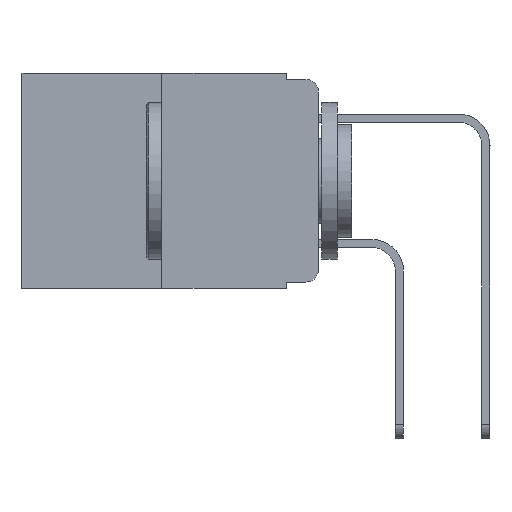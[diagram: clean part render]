
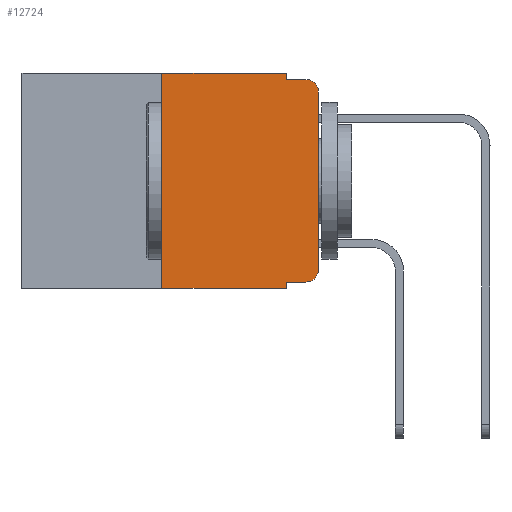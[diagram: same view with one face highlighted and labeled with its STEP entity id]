
A CAD part, left-side view. The second image highlights one B-rep face of the part: STEP entity #12724.
In plain terms, the highlighted planar face has unit normal (-1, 0, 0).
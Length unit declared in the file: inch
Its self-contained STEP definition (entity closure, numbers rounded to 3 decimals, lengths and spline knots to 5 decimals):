
#627 = LINE ( 'NONE', #11307, #21757 ) ;
#1274 = VERTEX_POINT ( 'NONE', #8650 ) ;
#1447 = VECTOR ( 'NONE', #20146, 39.37008 ) ;
#1574 = EDGE_CURVE ( 'NONE', #1274, #16716, #19780, .T. ) ;
#1789 = ORIENTED_EDGE ( 'NONE', *, *, #14009, .F. ) ;
#2052 = FACE_OUTER_BOUND ( 'NONE', #8509, .T. ) ;
#2379 = DIRECTION ( 'NONE',  ( 0., -1., 0. ) ) ;
#2404 = VECTOR ( 'NONE', #9807, 39.37008 ) ;
#2467 = LINE ( 'NONE', #9167, #5246 ) ;
#3691 = VERTEX_POINT ( 'NONE', #8519 ) ;
#4046 = VECTOR ( 'NONE', #21586, 39.37008 ) ;
#4500 = VECTOR ( 'NONE', #20394, 39.37008 ) ;
#4790 = VERTEX_POINT ( 'NONE', #8378 ) ;
#4875 = CARTESIAN_POINT ( 'NONE',  ( 0., 0.25, 0. ) ) ;
#5116 = ORIENTED_EDGE ( 'NONE', *, *, #1574, .T. ) ;
#5246 = VECTOR ( 'NONE', #16321, 39.37008 ) ;
#5424 = ORIENTED_EDGE ( 'NONE', *, *, #16774, .T. ) ;
#5484 = CARTESIAN_POINT ( 'NONE',  ( 0., 0.02, -0.03 ) ) ;
#6017 = LINE ( 'NONE', #20479, #2404 ) ;
#6065 = CARTESIAN_POINT ( 'NONE',  ( 0., 0.02, -0.333 ) ) ;
#6272 = VECTOR ( 'NONE', #22217, 39.37008 ) ;
#7768 = AXIS2_PLACEMENT_3D ( 'NONE', #10038, #13633, #17211 ) ;
#7793 = CARTESIAN_POINT ( 'NONE',  ( 0., 0.473, -0.343 ) ) ;
#8199 = LINE ( 'NONE', #14960, #6272 ) ;
#8378 = CARTESIAN_POINT ( 'NONE',  ( 0., 0.051, 0. ) ) ;
#8495 = CARTESIAN_POINT ( 'NONE',  ( 0., 0.051, -0.343 ) ) ;
#8509 = EDGE_LOOP ( 'NONE', ( #22162, #5424, #14634, #11281, #1789, #23008, #5116, #17263, #17312, #12977 ) ) ;
#8519 = CARTESIAN_POINT ( 'NONE',  ( 0., 0., -0.313 ) ) ;
#8650 = CARTESIAN_POINT ( 'NONE',  ( 0., 0.25, -0.343 ) ) ;
#8924 = LINE ( 'NONE', #17267, #1447 ) ;
#9161 = CARTESIAN_POINT ( 'NONE',  ( 0., 0.051, -0.01 ) ) ;
#9167 = CARTESIAN_POINT ( 'NONE',  ( 0., 0.051, -0.333 ) ) ;
#9543 = EDGE_CURVE ( 'NONE', #1274, #20126, #17157, .T. ) ;
#9807 = DIRECTION ( 'NONE',  ( 0., 0., 1. ) ) ;
#10038 = CARTESIAN_POINT ( 'NONE',  ( 0., 0.02, -0.313 ) ) ;
#10451 = CIRCLE ( 'NONE', #22774, 0.02 ) ;
#10657 = LINE ( 'NONE', #12635, #4046 ) ;
#10987 = EDGE_CURVE ( 'NONE', #13786, #16716, #10657, .T. ) ;
#11281 = ORIENTED_EDGE ( 'NONE', *, *, #17051, .F. ) ;
#11307 = CARTESIAN_POINT ( 'NONE',  ( 0., 0.051, -0.01 ) ) ;
#11659 = EDGE_CURVE ( 'NONE', #13728, #3691, #20128, .T. ) ;
#11779 = CARTESIAN_POINT ( 'NONE',  ( 0., 0.02, -0.01 ) ) ;
#12148 = VECTOR ( 'NONE', #13687, 39.37008 ) ;
#12386 = DIRECTION ( 'NONE',  ( 0., 0., -1. ) ) ;
#12558 = CARTESIAN_POINT ( 'NONE',  ( 0., 0.051, -0.333 ) ) ;
#12615 = DIRECTION ( 'NONE',  ( -1., 0., 0. ) ) ;
#12635 = CARTESIAN_POINT ( 'NONE',  ( 0., 0.051, 0. ) ) ;
#12724 = ADVANCED_FACE ( 'NONE', ( #2052 ), #13931, .F. ) ;
#12977 = ORIENTED_EDGE ( 'NONE', *, *, #11659, .T. ) ;
#13442 = AXIS2_PLACEMENT_3D ( 'NONE', #22747, #19292, #19154 ) ;
#13633 = DIRECTION ( 'NONE',  ( -1., 0., 0. ) ) ;
#13687 = DIRECTION ( 'NONE',  ( 0., 0., 1. ) ) ;
#13728 = VERTEX_POINT ( 'NONE', #6065 ) ;
#13786 = VERTEX_POINT ( 'NONE', #12558 ) ;
#13931 = PLANE ( 'NONE',  #13442 ) ;
#14009 = EDGE_CURVE ( 'NONE', #20126, #4790, #8924, .T. ) ;
#14183 = EDGE_CURVE ( 'NONE', #20949, #18418, #627, .T. ) ;
#14634 = ORIENTED_EDGE ( 'NONE', *, *, #14183, .F. ) ;
#14960 = CARTESIAN_POINT ( 'NONE',  ( 0., 0.051, 0. ) ) ;
#15647 = EDGE_CURVE ( 'NONE', #13786, #13728, #2467, .T. ) ;
#16321 = DIRECTION ( 'NONE',  ( 0., -1., 0. ) ) ;
#16716 = VERTEX_POINT ( 'NONE', #8495 ) ;
#16774 = EDGE_CURVE ( 'NONE', #17766, #18418, #10451, .T. ) ;
#16794 = CARTESIAN_POINT ( 'NONE',  ( 0., 0., -0.03 ) ) ;
#17051 = EDGE_CURVE ( 'NONE', #4790, #20949, #8199, .T. ) ;
#17157 = LINE ( 'NONE', #17261, #12148 ) ;
#17211 = DIRECTION ( 'NONE',  ( 0., 0., -1. ) ) ;
#17261 = CARTESIAN_POINT ( 'NONE',  ( 0., 0.25, 0. ) ) ;
#17263 = ORIENTED_EDGE ( 'NONE', *, *, #10987, .F. ) ;
#17267 = CARTESIAN_POINT ( 'NONE',  ( 0., 0.473, 0. ) ) ;
#17312 = ORIENTED_EDGE ( 'NONE', *, *, #15647, .T. ) ;
#17766 = VERTEX_POINT ( 'NONE', #16794 ) ;
#18418 = VERTEX_POINT ( 'NONE', #11779 ) ;
#19154 = DIRECTION ( 'NONE',  ( 0., 0., -1. ) ) ;
#19292 = DIRECTION ( 'NONE',  ( 1., 0., 0. ) ) ;
#19780 = LINE ( 'NONE', #7793, #4500 ) ;
#20047 = EDGE_CURVE ( 'NONE', #3691, #17766, #6017, .T. ) ;
#20126 = VERTEX_POINT ( 'NONE', #4875 ) ;
#20128 = CIRCLE ( 'NONE', #7768, 0.02 ) ;
#20146 = DIRECTION ( 'NONE',  ( 0., -1., 0. ) ) ;
#20394 = DIRECTION ( 'NONE',  ( 0., -1., 0. ) ) ;
#20479 = CARTESIAN_POINT ( 'NONE',  ( 0., 0., 0. ) ) ;
#20949 = VERTEX_POINT ( 'NONE', #9161 ) ;
#21586 = DIRECTION ( 'NONE',  ( 0., 0., -1. ) ) ;
#21757 = VECTOR ( 'NONE', #2379, 39.37008 ) ;
#22162 = ORIENTED_EDGE ( 'NONE', *, *, #20047, .T. ) ;
#22217 = DIRECTION ( 'NONE',  ( 0., 0., -1. ) ) ;
#22747 = CARTESIAN_POINT ( 'NONE',  ( 0., 0.473, 0. ) ) ;
#22774 = AXIS2_PLACEMENT_3D ( 'NONE', #5484, #12615, #12386 ) ;
#23008 = ORIENTED_EDGE ( 'NONE', *, *, #9543, .F. ) ;
